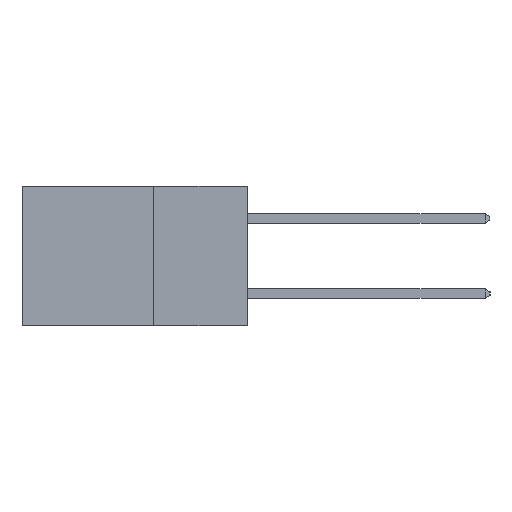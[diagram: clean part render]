
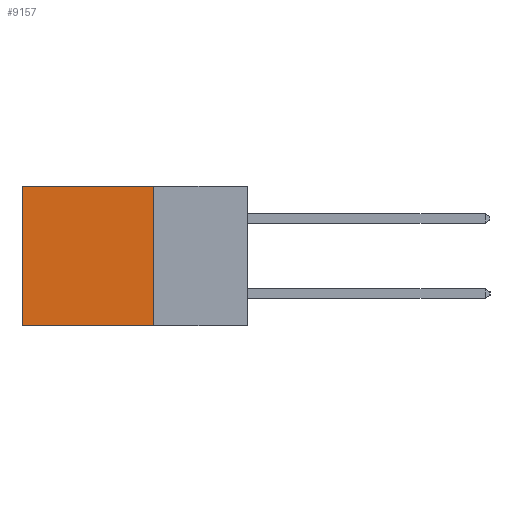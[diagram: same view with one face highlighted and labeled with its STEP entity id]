
A CAD part, left-side view. The second image highlights one B-rep face of the part: STEP entity #9157.
In plain terms, the highlighted planar face has unit normal (-1, 0, 0).
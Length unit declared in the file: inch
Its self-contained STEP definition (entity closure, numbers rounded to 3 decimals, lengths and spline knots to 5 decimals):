
#93 = ORIENTED_EDGE ( 'NONE', *, *, #10630, .T. ) ;
#1301 = DIRECTION ( 'NONE',  ( 0., 0., -1. ) ) ;
#1353 = CARTESIAN_POINT ( 'NONE',  ( 0.2615, 0.25, -0.37 ) ) ;
#2226 = CARTESIAN_POINT ( 'NONE',  ( 0.2615, 0.25, -0.37 ) ) ;
#2565 = LINE ( 'NONE', #1353, #11197 ) ;
#2875 = VERTEX_POINT ( 'NONE', #5026 ) ;
#2972 = DIRECTION ( 'NONE',  ( 0., 1., 0. ) ) ;
#3062 = EDGE_CURVE ( 'NONE', #5351, #13877, #2565, .T. ) ;
#3209 = CARTESIAN_POINT ( 'NONE',  ( 0.2615, 0.6, -0.37 ) ) ;
#3232 = DIRECTION ( 'NONE',  ( 0., 0., -1. ) ) ;
#3252 = DIRECTION ( 'NONE',  ( 1., 0., 0. ) ) ;
#3284 = PLANE ( 'NONE',  #3594 ) ;
#3538 = CARTESIAN_POINT ( 'NONE',  ( 0.2615, 0.25, -0.37 ) ) ;
#3594 = AXIS2_PLACEMENT_3D ( 'NONE', #3538, #3252, #3232 ) ;
#3855 = CARTESIAN_POINT ( 'NONE',  ( 0.2615, 0.25, 0. ) ) ;
#3983 = ORIENTED_EDGE ( 'NONE', *, *, #13590, .F. ) ;
#4015 = VECTOR ( 'NONE', #11069, 39.37008 ) ;
#4173 = VERTEX_POINT ( 'NONE', #12052 ) ;
#5026 = CARTESIAN_POINT ( 'NONE',  ( 0.2615, 0.6, 0. ) ) ;
#5035 = FACE_OUTER_BOUND ( 'NONE', #13151, .T. ) ;
#5176 = DIRECTION ( 'NONE',  ( 0., 1., 0. ) ) ;
#5351 = VERTEX_POINT ( 'NONE', #3855 ) ;
#6423 = CARTESIAN_POINT ( 'NONE',  ( 0.2615, 0.25, 0. ) ) ;
#6806 = ORIENTED_EDGE ( 'NONE', *, *, #3062, .F. ) ;
#7092 = LINE ( 'NONE', #3209, #4015 ) ;
#8571 = CARTESIAN_POINT ( 'NONE',  ( 0.2615, 0.25, -0.37 ) ) ;
#8909 = VECTOR ( 'NONE', #2972, 39.37008 ) ;
#9013 = VECTOR ( 'NONE', #5176, 39.37008 ) ;
#9157 = ADVANCED_FACE ( 'NONE', ( #5035 ), #3284, .F. ) ;
#10630 = EDGE_CURVE ( 'NONE', #5351, #2875, #11769, .T. ) ;
#11069 = DIRECTION ( 'NONE',  ( 0., 0., -1. ) ) ;
#11197 = VECTOR ( 'NONE', #1301, 39.37008 ) ;
#11685 = ORIENTED_EDGE ( 'NONE', *, *, #13116, .T. ) ;
#11769 = LINE ( 'NONE', #6423, #8909 ) ;
#11865 = LINE ( 'NONE', #8571, #9013 ) ;
#12052 = CARTESIAN_POINT ( 'NONE',  ( 0.2615, 0.6, -0.37 ) ) ;
#13116 = EDGE_CURVE ( 'NONE', #2875, #4173, #7092, .T. ) ;
#13151 = EDGE_LOOP ( 'NONE', ( #11685, #3983, #6806, #93 ) ) ;
#13590 = EDGE_CURVE ( 'NONE', #13877, #4173, #11865, .T. ) ;
#13877 = VERTEX_POINT ( 'NONE', #2226 ) ;
